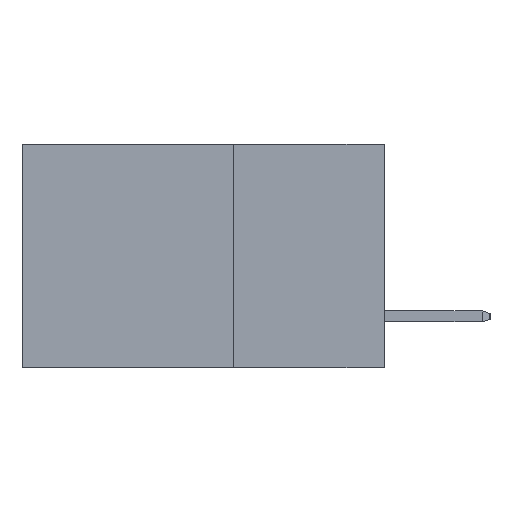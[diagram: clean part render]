
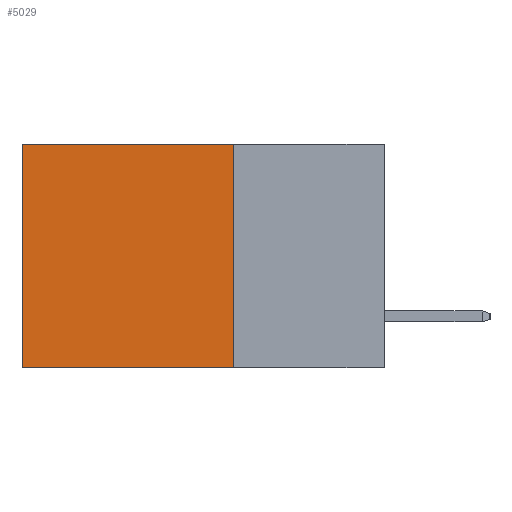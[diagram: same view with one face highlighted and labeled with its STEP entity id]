
A CAD part, left-side view. The second image highlights one B-rep face of the part: STEP entity #5029.
In plain terms, the highlighted planar face has unit normal (-1, 0, 0).
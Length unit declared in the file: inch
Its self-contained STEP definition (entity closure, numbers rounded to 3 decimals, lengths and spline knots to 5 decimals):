
#17 = FACE_OUTER_BOUND ( 'NONE', #7203, .T. ) ;
#709 = CARTESIAN_POINT ( 'NONE',  ( 0.2615, 0.6, 0. ) ) ;
#1866 = VECTOR ( 'NONE', #10997, 39.37008 ) ;
#2572 = VECTOR ( 'NONE', #11163, 39.37008 ) ;
#2845 = CARTESIAN_POINT ( 'NONE',  ( 0.2615, 0.6, -0.37 ) ) ;
#3729 = CARTESIAN_POINT ( 'NONE',  ( 0.2615, 0.25, 0. ) ) ;
#4157 = VECTOR ( 'NONE', #7974, 39.37008 ) ;
#5029 = ADVANCED_FACE ( 'NONE', ( #17 ), #11191, .F. ) ;
#5148 = LINE ( 'NONE', #2845, #2572 ) ;
#5537 = ORIENTED_EDGE ( 'NONE', *, *, #6016, .F. ) ;
#5726 = ORIENTED_EDGE ( 'NONE', *, *, #10320, .F. ) ;
#5950 = ORIENTED_EDGE ( 'NONE', *, *, #7172, .T. ) ;
#6016 = EDGE_CURVE ( 'NONE', #6286, #11279, #11465, .T. ) ;
#6286 = VERTEX_POINT ( 'NONE', #3729 ) ;
#7030 = LINE ( 'NONE', #10186, #1866 ) ;
#7162 = ORIENTED_EDGE ( 'NONE', *, *, #9746, .T. ) ;
#7172 = EDGE_CURVE ( 'NONE', #8654, #8857, #5148, .T. ) ;
#7203 = EDGE_LOOP ( 'NONE', ( #5950, #5726, #5537, #7162 ) ) ;
#7435 = CARTESIAN_POINT ( 'NONE',  ( 0.2615, 0.25, -0.37 ) ) ;
#7720 = LINE ( 'NONE', #7435, #12126 ) ;
#7974 = DIRECTION ( 'NONE',  ( 0., 0., -1. ) ) ;
#8386 = DIRECTION ( 'NONE',  ( 0., 1., 0. ) ) ;
#8448 = AXIS2_PLACEMENT_3D ( 'NONE', #11367, #10690, #10676 ) ;
#8497 = CARTESIAN_POINT ( 'NONE',  ( 0.2615, 0.25, -0.37 ) ) ;
#8539 = CARTESIAN_POINT ( 'NONE',  ( 0.2615, 0.25, -0.37 ) ) ;
#8654 = VERTEX_POINT ( 'NONE', #709 ) ;
#8857 = VERTEX_POINT ( 'NONE', #11460 ) ;
#9746 = EDGE_CURVE ( 'NONE', #6286, #8654, #7030, .T. ) ;
#10186 = CARTESIAN_POINT ( 'NONE',  ( 0.2615, 0.25, 0. ) ) ;
#10320 = EDGE_CURVE ( 'NONE', #11279, #8857, #7720, .T. ) ;
#10676 = DIRECTION ( 'NONE',  ( 0., 0., -1. ) ) ;
#10690 = DIRECTION ( 'NONE',  ( 1., 0., 0. ) ) ;
#10997 = DIRECTION ( 'NONE',  ( 0., 1., 0. ) ) ;
#11163 = DIRECTION ( 'NONE',  ( 0., 0., -1. ) ) ;
#11191 = PLANE ( 'NONE',  #8448 ) ;
#11279 = VERTEX_POINT ( 'NONE', #8539 ) ;
#11367 = CARTESIAN_POINT ( 'NONE',  ( 0.2615, 0.25, -0.37 ) ) ;
#11460 = CARTESIAN_POINT ( 'NONE',  ( 0.2615, 0.6, -0.37 ) ) ;
#11465 = LINE ( 'NONE', #8497, #4157 ) ;
#12126 = VECTOR ( 'NONE', #8386, 39.37008 ) ;
